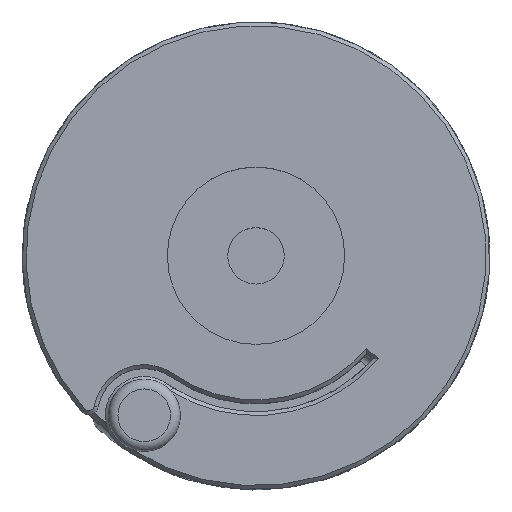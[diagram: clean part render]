
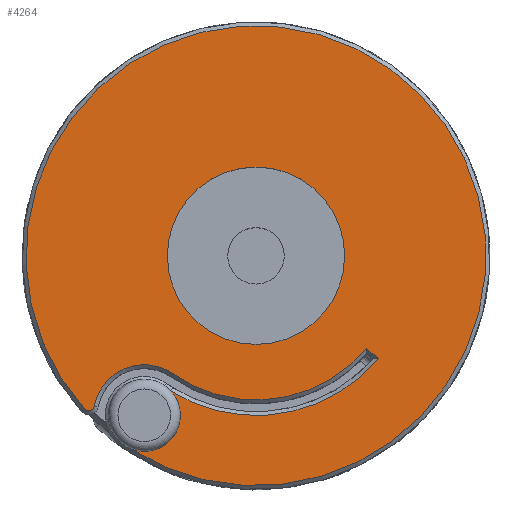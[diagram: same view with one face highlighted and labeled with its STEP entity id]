
A CAD part, top view. The second image highlights one B-rep face of the part: STEP entity #4264.
In plain terms, the highlighted planar face has unit normal (0, 0, 1).
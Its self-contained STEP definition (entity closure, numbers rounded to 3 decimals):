
#19=FACE_BOUND('',#1156,.T.);
#173=PLANE('',#4657);
#431=LINE('',#6122,#559);
#559=VECTOR('',#5006,10.);
#854=FACE_OUTER_BOUND('',#1155,.T.);
#1155=EDGE_LOOP('',(#3127,#3128,#3129,#3130,#3131,#3132,#3133,#3134));
#1156=EDGE_LOOP('',(#3135));
#1386=CIRCLE('',#4509,1.85);
#1387=CIRCLE('',#4510,1.85);
#1389=CIRCLE('',#4516,2.6);
#1392=CIRCLE('',#4520,0.3);
#1393=CIRCLE('',#4522,7.4);
#1397=CIRCLE('',#4529,11.8);
#1475=CIRCLE('',#4650,4.55);
#1477=CIRCLE('',#4653,8.2);
#1689=VERTEX_POINT('',#6074);
#1690=VERTEX_POINT('',#6075);
#1691=VERTEX_POINT('',#6078);
#1694=VERTEX_POINT('',#6111);
#1697=VERTEX_POINT('',#6118);
#1704=VERTEX_POINT('',#6150);
#1705=VERTEX_POINT('',#6152);
#1708=VERTEX_POINT('',#6159);
#1821=VERTEX_POINT('',#7308);
#2088=EDGE_CURVE('',#1689,#1690,#1386,.T.);
#2090=EDGE_CURVE('',#1690,#1691,#1387,.T.);
#2097=EDGE_CURVE('',#1697,#1694,#431,.T.);
#2105=EDGE_CURVE('',#1704,#1705,#1389,.T.);
#2110=EDGE_CURVE('',#1705,#1708,#1392,.T.);
#2111=EDGE_CURVE('',#1694,#1704,#1393,.T.);
#2121=EDGE_CURVE('',#1708,#1689,#1397,.T.);
#2281=EDGE_CURVE('',#1821,#1821,#1475,.T.);
#2285=EDGE_CURVE('',#1691,#1697,#1477,.T.);
#3127=ORIENTED_EDGE('',*,*,#2285,.F.);
#3128=ORIENTED_EDGE('',*,*,#2090,.F.);
#3129=ORIENTED_EDGE('',*,*,#2088,.F.);
#3130=ORIENTED_EDGE('',*,*,#2121,.F.);
#3131=ORIENTED_EDGE('',*,*,#2110,.F.);
#3132=ORIENTED_EDGE('',*,*,#2105,.F.);
#3133=ORIENTED_EDGE('',*,*,#2111,.F.);
#3134=ORIENTED_EDGE('',*,*,#2097,.F.);
#3135=ORIENTED_EDGE('',*,*,#2281,.T.);
#4264=ADVANCED_FACE('',(#854,#19),#173,.F.);
#4509=AXIS2_PLACEMENT_3D('',#6076,#4994,#4995);
#4510=AXIS2_PLACEMENT_3D('',#6079,#4997,#4998);
#4516=AXIS2_PLACEMENT_3D('',#6153,#5017,#5018);
#4520=AXIS2_PLACEMENT_3D('',#6162,#5027,#5028);
#4522=AXIS2_PLACEMENT_3D('',#6164,#5031,#5032);
#4529=AXIS2_PLACEMENT_3D('',#6201,#5048,#5049);
#4650=AXIS2_PLACEMENT_3D('',#7309,#5324,#5325);
#4653=AXIS2_PLACEMENT_3D('',#7316,#5332,#5333);
#4657=AXIS2_PLACEMENT_3D('',#7359,#5342,#5343);
#4994=DIRECTION('center_axis',(0.,0.,1.));
#4995=DIRECTION('ref_axis',(0.,1.,0.));
#4997=DIRECTION('center_axis',(0.,0.,1.));
#4998=DIRECTION('ref_axis',(0.,1.,0.));
#5006=DIRECTION('',(-0.749,0.663,0.));
#5017=DIRECTION('center_axis',(0.,0.,1.));
#5018=DIRECTION('ref_axis',(0.,1.,0.));
#5027=DIRECTION('center_axis',(0.,0.,-1.));
#5028=DIRECTION('ref_axis',(0.267,-0.964,0.));
#5031=DIRECTION('center_axis',(0.,0.,-1.));
#5032=DIRECTION('ref_axis',(0.,-1.,0.));
#5048=DIRECTION('center_axis',(0.,0.,-1.));
#5049=DIRECTION('ref_axis',(0.,1.,0.));
#5324=DIRECTION('center_axis',(0.,0.,-1.));
#5325=DIRECTION('ref_axis',(0.,1.,0.));
#5332=DIRECTION('center_axis',(0.,0.,1.));
#5333=DIRECTION('ref_axis',(0.,-1.,0.));
#5342=DIRECTION('center_axis',(0.,0.,-1.));
#5343=DIRECTION('ref_axis',(0.,-1.,0.));
#6074=CARTESIAN_POINT('',(-127.683,-20.625,14.8));
#6075=CARTESIAN_POINT('',(-127.036,-20.742,14.8));
#6076=CARTESIAN_POINT('Origin',(-127.036,-18.892,14.8));
#6078=CARTESIAN_POINT('',(-125.681,-17.631,14.8));
#6079=CARTESIAN_POINT('Origin',(-127.036,-18.892,14.8));
#6111=CARTESIAN_POINT('',(-115.627,-15.451,14.8));
#6118=CARTESIAN_POINT('',(-115.027,-15.981,14.8));
#6122=CARTESIAN_POINT('',(-118.323,-13.066,14.8));
#6150=CARTESIAN_POINT('',(-125.544,-16.762,14.8));
#6152=CARTESIAN_POINT('',(-129.59,-18.407,14.8));
#6153=CARTESIAN_POINT('Origin',(-127.036,-18.892,14.8));
#6159=CARTESIAN_POINT('',(-130.109,-18.551,14.8));
#6162=CARTESIAN_POINT('Origin',(-129.885,-18.352,14.8));
#6164=CARTESIAN_POINT('Origin',(-121.3,-10.7,14.8));
#6201=CARTESIAN_POINT('Origin',(-121.3,-10.7,14.8));
#7308=CARTESIAN_POINT('',(-121.3,-15.25,14.8));
#7309=CARTESIAN_POINT('Origin',(-121.3,-10.7,14.8));
#7316=CARTESIAN_POINT('Origin',(-121.3,-10.7,14.8));
#7359=CARTESIAN_POINT('Origin',(-121.573,-10.7,14.8));
